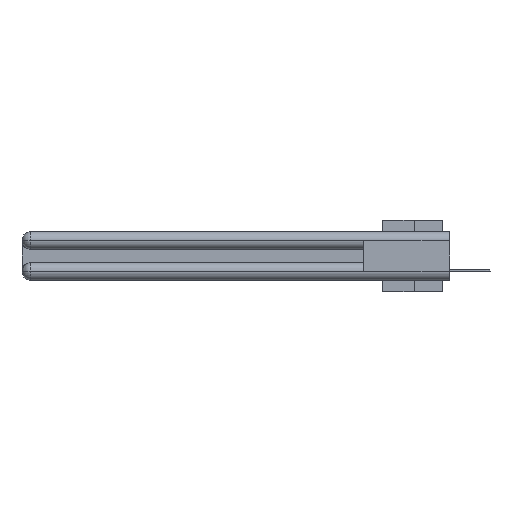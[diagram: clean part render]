
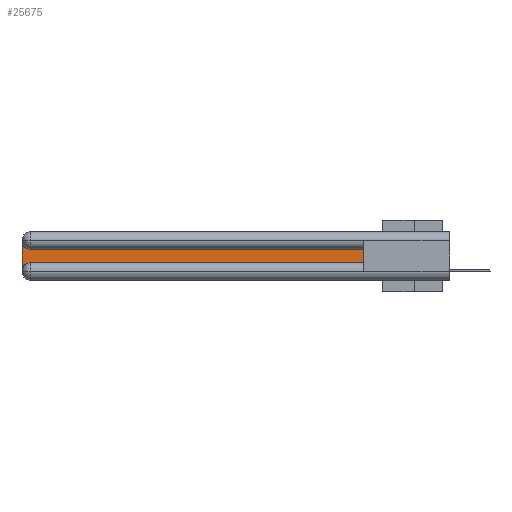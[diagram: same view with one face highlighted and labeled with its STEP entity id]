
A CAD part, left-side view. The second image highlights one B-rep face of the part: STEP entity #25675.
In plain terms, the highlighted planar face has unit normal (-1, 0, 0).
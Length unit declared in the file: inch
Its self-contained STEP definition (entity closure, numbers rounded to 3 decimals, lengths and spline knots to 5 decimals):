
#863 = AXIS2_PLACEMENT_3D ( 'NONE', #22009, #16874, #12116 ) ;
#1009 = DIRECTION ( 'NONE',  ( 1., 0., 0. ) ) ;
#1021 = VECTOR ( 'NONE', #17633, 39.37008 ) ;
#1182 = ORIENTED_EDGE ( 'NONE', *, *, #12372, .T. ) ;
#1447 = DIRECTION ( 'NONE',  ( 0., 0., -1. ) ) ;
#1743 = ORIENTED_EDGE ( 'NONE', *, *, #10456, .T. ) ;
#2046 = VERTEX_POINT ( 'NONE', #30021 ) ;
#2798 = VERTEX_POINT ( 'NONE', #14014 ) ;
#3304 = VERTEX_POINT ( 'NONE', #28469 ) ;
#4037 = EDGE_CURVE ( 'NONE', #23746, #2798, #25027, .T. ) ;
#4996 = EDGE_LOOP ( 'NONE', ( #29946, #11475, #10867, #1743, #9022, #1182 ) ) ;
#5236 = DIRECTION ( 'NONE',  ( 0., 0., -1. ) ) ;
#5342 = VERTEX_POINT ( 'NONE', #24232 ) ;
#6296 = VECTOR ( 'NONE', #11759, 39.37008 ) ;
#6764 = CARTESIAN_POINT ( 'NONE',  ( 0.075, 2.94, -0.2775 ) ) ;
#7557 = LINE ( 'NONE', #27643, #1021 ) ;
#8155 = LINE ( 'NONE', #26936, #6296 ) ;
#8322 = CIRCLE ( 'NONE', #18501, 0.06 ) ;
#9022 = ORIENTED_EDGE ( 'NONE', *, *, #24052, .T. ) ;
#9208 = DIRECTION ( 'NONE',  ( 1., 0., 0. ) ) ;
#10456 = EDGE_CURVE ( 'NONE', #2046, #5342, #8322, .T. ) ;
#10867 = ORIENTED_EDGE ( 'NONE', *, *, #16150, .T. ) ;
#11179 = CARTESIAN_POINT ( 'NONE',  ( 0.075, 0.6, -0.1225 ) ) ;
#11185 = FACE_OUTER_BOUND ( 'NONE', #4996, .T. ) ;
#11475 = ORIENTED_EDGE ( 'NONE', *, *, #4037, .T. ) ;
#11759 = DIRECTION ( 'NONE',  ( 0., 0., 1. ) ) ;
#12116 = DIRECTION ( 'NONE',  ( 0., 0., -1. ) ) ;
#12167 = VERTEX_POINT ( 'NONE', #11179 ) ;
#12372 = EDGE_CURVE ( 'NONE', #3304, #12167, #8155, .T. ) ;
#12931 = CARTESIAN_POINT ( 'NONE',  ( 0.075, 3., -0.2175 ) ) ;
#13174 = AXIS2_PLACEMENT_3D ( 'NONE', #26194, #1009, #1447 ) ;
#13275 = LINE ( 'NONE', #12931, #16389 ) ;
#14014 = CARTESIAN_POINT ( 'NONE',  ( 0.075, 3., -0.0625 ) ) ;
#14136 = DIRECTION ( 'NONE',  ( 0., 0., -1. ) ) ;
#16150 = EDGE_CURVE ( 'NONE', #2798, #2046, #13275, .T. ) ;
#16389 = VECTOR ( 'NONE', #5236, 39.37008 ) ;
#16874 = DIRECTION ( 'NONE',  ( 1., 0., 0. ) ) ;
#17271 = DIRECTION ( 'NONE',  ( 0., -1., 0. ) ) ;
#17633 = DIRECTION ( 'NONE',  ( 0., 1., 0. ) ) ;
#18501 = AXIS2_PLACEMENT_3D ( 'NONE', #6764, #9208, #14136 ) ;
#19796 = LINE ( 'NONE', #22306, #23757 ) ;
#21954 = EDGE_CURVE ( 'NONE', #12167, #23746, #7557, .T. ) ;
#22009 = CARTESIAN_POINT ( 'NONE',  ( 0.075, 3., -0.1225 ) ) ;
#22306 = CARTESIAN_POINT ( 'NONE',  ( 0.075, 0.6, -0.2175 ) ) ;
#23746 = VERTEX_POINT ( 'NONE', #31302 ) ;
#23757 = VECTOR ( 'NONE', #17271, 39.37008 ) ;
#24052 = EDGE_CURVE ( 'NONE', #5342, #3304, #19796, .T. ) ;
#24232 = CARTESIAN_POINT ( 'NONE',  ( 0.075, 2.94, -0.2175 ) ) ;
#25027 = CIRCLE ( 'NONE', #13174, 0.06 ) ;
#25675 = ADVANCED_FACE ( 'NONE', ( #11185 ), #31725, .F. ) ;
#26194 = CARTESIAN_POINT ( 'NONE',  ( 0.075, 2.94, -0.0625 ) ) ;
#26936 = CARTESIAN_POINT ( 'NONE',  ( 0.075, 0.6, -0.2175 ) ) ;
#27643 = CARTESIAN_POINT ( 'NONE',  ( 0.075, 0.6, -0.1225 ) ) ;
#28469 = CARTESIAN_POINT ( 'NONE',  ( 0.075, 0.6, -0.2175 ) ) ;
#29946 = ORIENTED_EDGE ( 'NONE', *, *, #21954, .T. ) ;
#30021 = CARTESIAN_POINT ( 'NONE',  ( 0.075, 3., -0.2775 ) ) ;
#31302 = CARTESIAN_POINT ( 'NONE',  ( 0.075, 2.94, -0.1225 ) ) ;
#31725 = PLANE ( 'NONE',  #863 ) ;
